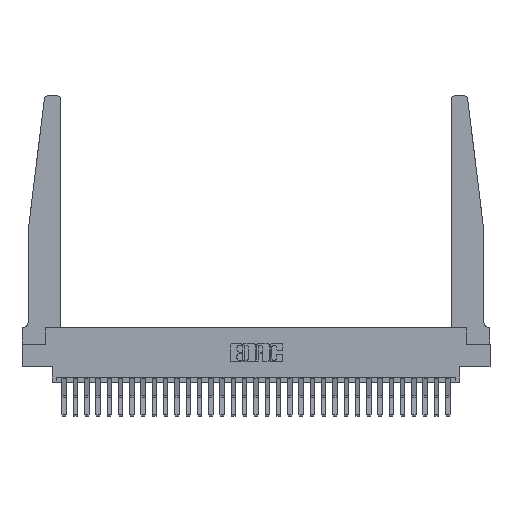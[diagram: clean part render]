
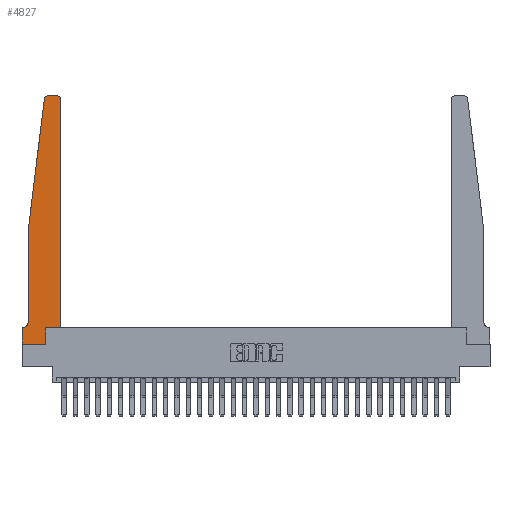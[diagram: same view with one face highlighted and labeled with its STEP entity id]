
A CAD part, top view. The second image highlights one B-rep face of the part: STEP entity #4827.
In plain terms, the highlighted planar face has unit normal (0, 0, 1).
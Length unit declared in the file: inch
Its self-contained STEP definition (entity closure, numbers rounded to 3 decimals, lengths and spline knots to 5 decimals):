
#478 = CARTESIAN_POINT ( 'NONE',  ( 0.2605, 0., 0.37 ) ) ;
#517 = VERTEX_POINT ( 'NONE', #5037 ) ;
#520 = FACE_OUTER_BOUND ( 'NONE', #1286, .T. ) ;
#1215 = AXIS2_PLACEMENT_3D ( 'NONE', #2622, #25070, #26871 ) ;
#1286 = EDGE_LOOP ( 'NONE', ( #12930, #28110, #20827, #15576, #6247, #4558, #12333, #8058, #11299, #26417, #2383, #5302 ) ) ;
#1369 = CARTESIAN_POINT ( 'NONE',  ( 0.395, 2.72, 0.37 ) ) ;
#2062 = CIRCLE ( 'NONE', #8660, 0.05 ) ;
#2097 = DIRECTION ( 'NONE',  ( 0., -1., 0. ) ) ;
#2383 = ORIENTED_EDGE ( 'NONE', *, *, #7140, .T. ) ;
#2622 = CARTESIAN_POINT ( 'NONE',  ( 0.27653, 2.72, 0.37 ) ) ;
#2787 = AXIS2_PLACEMENT_3D ( 'NONE', #14114, #23257, #20457 ) ;
#3133 = CIRCLE ( 'NONE', #1215, 0.03 ) ;
#3706 = VECTOR ( 'NONE', #5047, 39.37008 ) ;
#3720 = DIRECTION ( 'NONE',  ( 1., 0., 0. ) ) ;
#4017 = CARTESIAN_POINT ( 'NONE',  ( 0.065, 1.25, 0.37 ) ) ;
#4412 = CARTESIAN_POINT ( 'NONE',  ( 0.24675, 2.72367, 0.37 ) ) ;
#4558 = ORIENTED_EDGE ( 'NONE', *, *, #25893, .T. ) ;
#4827 = ADVANCED_FACE ( 'NONE', ( #520 ), #18810, .T. ) ;
#5037 = CARTESIAN_POINT ( 'NONE',  ( 0.425, 0.18, 0.37 ) ) ;
#5047 = DIRECTION ( 'NONE',  ( 1., 0., 0. ) ) ;
#5302 = ORIENTED_EDGE ( 'NONE', *, *, #17673, .T. ) ;
#5382 = VERTEX_POINT ( 'NONE', #24679 ) ;
#5464 = DIRECTION ( 'NONE',  ( -0.122, -0.992, 0. ) ) ;
#6174 = AXIS2_PLACEMENT_3D ( 'NONE', #1369, #21589, #3720 ) ;
#6247 = ORIENTED_EDGE ( 'NONE', *, *, #20810, .T. ) ;
#6736 = VECTOR ( 'NONE', #5464, 39.37008 ) ;
#7140 = EDGE_CURVE ( 'NONE', #517, #17167, #10781, .T. ) ;
#7313 = DIRECTION ( 'NONE',  ( -1., 0., 0. ) ) ;
#7479 = VERTEX_POINT ( 'NONE', #10864 ) ;
#7758 = VERTEX_POINT ( 'NONE', #16558 ) ;
#8058 = ORIENTED_EDGE ( 'NONE', *, *, #15072, .T. ) ;
#8419 = CARTESIAN_POINT ( 'NONE',  ( 0.425, 0.18, 0.37 ) ) ;
#8660 = AXIS2_PLACEMENT_3D ( 'NONE', #15368, #10952, #19939 ) ;
#9146 = CARTESIAN_POINT ( 'NONE',  ( 0.065, 1.25, 0.37 ) ) ;
#9555 = VERTEX_POINT ( 'NONE', #24962 ) ;
#9658 = LINE ( 'NONE', #16429, #21334 ) ;
#9672 = CARTESIAN_POINT ( 'NONE',  ( 0.065, 0.1875, 0.37 ) ) ;
#9955 = DIRECTION ( 'NONE',  ( 0., 1., 0. ) ) ;
#10078 = EDGE_CURVE ( 'NONE', #14968, #13417, #19356, .T. ) ;
#10781 = LINE ( 'NONE', #8419, #16905 ) ;
#10864 = CARTESIAN_POINT ( 'NONE',  ( 0., 0.1875, 0.37 ) ) ;
#10952 = DIRECTION ( 'NONE',  ( 0., 0., -1. ) ) ;
#11238 = EDGE_CURVE ( 'NONE', #5382, #28893, #3133, .T. ) ;
#11266 = CARTESIAN_POINT ( 'NONE',  ( 0., 0., 0.37 ) ) ;
#11299 = ORIENTED_EDGE ( 'NONE', *, *, #10078, .T. ) ;
#12333 = ORIENTED_EDGE ( 'NONE', *, *, #18938, .T. ) ;
#12725 = CARTESIAN_POINT ( 'NONE',  ( 0.2605, 0.18, 0.37 ) ) ;
#12930 = ORIENTED_EDGE ( 'NONE', *, *, #23717, .T. ) ;
#13295 = CARTESIAN_POINT ( 'NONE',  ( 0.065, 0.2375, 0.37 ) ) ;
#13417 = VERTEX_POINT ( 'NONE', #12725 ) ;
#14114 = CARTESIAN_POINT ( 'NONE',  ( 0., 0.1875, 0.37 ) ) ;
#14968 = VERTEX_POINT ( 'NONE', #478 ) ;
#15072 = EDGE_CURVE ( 'NONE', #7758, #14968, #22478, .T. ) ;
#15222 = VECTOR ( 'NONE', #20260, 39.37008 ) ;
#15368 = CARTESIAN_POINT ( 'NONE',  ( 0.015, 0.2375, 0.37 ) ) ;
#15483 = DIRECTION ( 'NONE',  ( 0., 1., 0. ) ) ;
#15576 = ORIENTED_EDGE ( 'NONE', *, *, #24862, .T. ) ;
#16429 = CARTESIAN_POINT ( 'NONE',  ( 0., 0., 0.37 ) ) ;
#16558 = CARTESIAN_POINT ( 'NONE',  ( 0., 0., 0.37 ) ) ;
#16564 = DIRECTION ( 'NONE',  ( 0., -1., 0. ) ) ;
#16635 = LINE ( 'NONE', #25699, #6736 ) ;
#16659 = LINE ( 'NONE', #25580, #3706 ) ;
#16905 = VECTOR ( 'NONE', #15483, 39.37008 ) ;
#17167 = VERTEX_POINT ( 'NONE', #18072 ) ;
#17465 = CIRCLE ( 'NONE', #6174, 0.03 ) ;
#17673 = EDGE_CURVE ( 'NONE', #17167, #24627, #17465, .T. ) ;
#17814 = VECTOR ( 'NONE', #9955, 39.37008 ) ;
#18072 = CARTESIAN_POINT ( 'NONE',  ( 0.425, 2.72, 0.37 ) ) ;
#18810 = PLANE ( 'NONE',  #2787 ) ;
#18938 = EDGE_CURVE ( 'NONE', #7479, #7758, #9658, .T. ) ;
#19207 = VERTEX_POINT ( 'NONE', #13295 ) ;
#19356 = LINE ( 'NONE', #28134, #17814 ) ;
#19726 = EDGE_CURVE ( 'NONE', #28893, #28909, #16635, .T. ) ;
#19939 = DIRECTION ( 'NONE',  ( -1., 0., 0. ) ) ;
#20102 = LINE ( 'NONE', #4017, #26705 ) ;
#20260 = DIRECTION ( 'NONE',  ( 1., 0., 0. ) ) ;
#20457 = DIRECTION ( 'NONE',  ( 1., 0., 0. ) ) ;
#20669 = DIRECTION ( 'NONE',  ( -1., 0., 0. ) ) ;
#20810 = EDGE_CURVE ( 'NONE', #19207, #9555, #2062, .T. ) ;
#20827 = ORIENTED_EDGE ( 'NONE', *, *, #19726, .T. ) ;
#21183 = LINE ( 'NONE', #9672, #23871 ) ;
#21334 = VECTOR ( 'NONE', #16564, 39.37008 ) ;
#21589 = DIRECTION ( 'NONE',  ( 0., 0., 1. ) ) ;
#22478 = LINE ( 'NONE', #11266, #15222 ) ;
#23257 = DIRECTION ( 'NONE',  ( 0., 0., 1. ) ) ;
#23304 = CARTESIAN_POINT ( 'NONE',  ( 0.25, 2.75, 0.37 ) ) ;
#23371 = VECTOR ( 'NONE', #20669, 39.37008 ) ;
#23717 = EDGE_CURVE ( 'NONE', #24627, #5382, #28063, .T. ) ;
#23871 = VECTOR ( 'NONE', #7313, 39.37008 ) ;
#23964 = CARTESIAN_POINT ( 'NONE',  ( 0.395, 2.75, 0.37 ) ) ;
#24627 = VERTEX_POINT ( 'NONE', #23964 ) ;
#24679 = CARTESIAN_POINT ( 'NONE',  ( 0.27653, 2.75, 0.37 ) ) ;
#24862 = EDGE_CURVE ( 'NONE', #28909, #19207, #20102, .T. ) ;
#24962 = CARTESIAN_POINT ( 'NONE',  ( 0.015, 0.1875, 0.37 ) ) ;
#25070 = DIRECTION ( 'NONE',  ( 0., 0., 1. ) ) ;
#25580 = CARTESIAN_POINT ( 'NONE',  ( 0.425, 0.18, 0.37 ) ) ;
#25699 = CARTESIAN_POINT ( 'NONE',  ( 0.065, 1.25, 0.37 ) ) ;
#25893 = EDGE_CURVE ( 'NONE', #9555, #7479, #21183, .T. ) ;
#26417 = ORIENTED_EDGE ( 'NONE', *, *, #28606, .T. ) ;
#26705 = VECTOR ( 'NONE', #2097, 39.37008 ) ;
#26871 = DIRECTION ( 'NONE',  ( 1., 0., 0. ) ) ;
#28063 = LINE ( 'NONE', #23304, #23371 ) ;
#28110 = ORIENTED_EDGE ( 'NONE', *, *, #11238, .T. ) ;
#28134 = CARTESIAN_POINT ( 'NONE',  ( 0.2605, 0.18, 0.37 ) ) ;
#28606 = EDGE_CURVE ( 'NONE', #13417, #517, #16659, .T. ) ;
#28893 = VERTEX_POINT ( 'NONE', #4412 ) ;
#28909 = VERTEX_POINT ( 'NONE', #9146 ) ;
